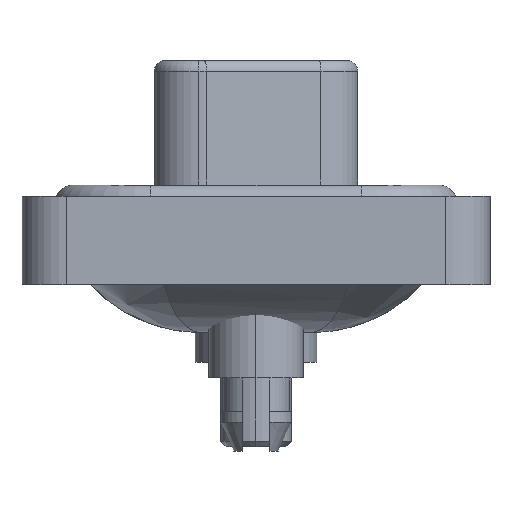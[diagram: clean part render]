
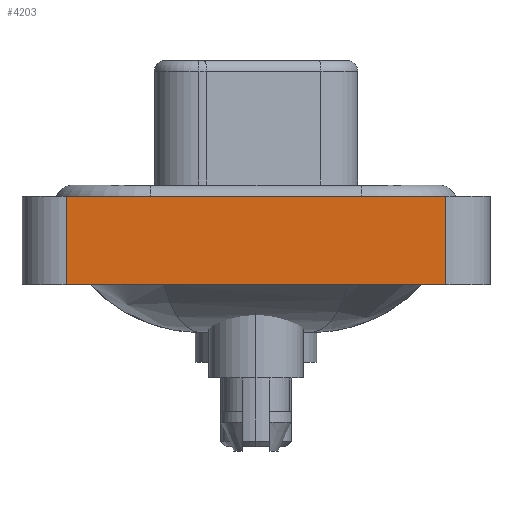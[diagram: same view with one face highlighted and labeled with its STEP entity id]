
A CAD part, left-side view. The second image highlights one B-rep face of the part: STEP entity #4203.
In plain terms, the highlighted planar face has unit normal (-1, 0, 0).
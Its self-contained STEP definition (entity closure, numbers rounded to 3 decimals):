
#140 = PLANE ( 'NONE',  #11697 ) ;
#316 = DIRECTION ( 'NONE',  ( 0., 0., 1. ) ) ;
#1077 = ORIENTED_EDGE ( 'NONE', *, *, #5960, .F. ) ;
#1085 = CARTESIAN_POINT ( 'NONE',  ( -7.3, -8.55, 0.4 ) ) ;
#1800 = VECTOR ( 'NONE', #1956, 1000. ) ;
#1956 = DIRECTION ( 'NONE',  ( 0., -1., 0. ) ) ;
#2335 = CARTESIAN_POINT ( 'NONE',  ( -7.3, -8.55, 0.4 ) ) ;
#3457 = EDGE_LOOP ( 'NONE', ( #10980, #4204, #1077, #15830 ) ) ;
#4203 = ADVANCED_FACE ( 'NONE', ( #16475 ), #140, .T. ) ;
#4204 = ORIENTED_EDGE ( 'NONE', *, *, #10672, .F. ) ;
#5868 = LINE ( 'NONE', #13966, #1800 ) ;
#5960 = EDGE_CURVE ( 'NONE', #15395, #13052, #7998, .T. ) ;
#6422 = DIRECTION ( 'NONE',  ( 0., -1., 0. ) ) ;
#6580 = CARTESIAN_POINT ( 'NONE',  ( -7.3, -8.55, -3.6 ) ) ;
#6786 = DIRECTION ( 'NONE',  ( -1., 0., 0. ) ) ;
#7095 = VERTEX_POINT ( 'NONE', #14334 ) ;
#7142 = CARTESIAN_POINT ( 'NONE',  ( -7.3, -8.55, -3.6 ) ) ;
#7898 = DIRECTION ( 'NONE',  ( 0., 0., 1. ) ) ;
#7998 = LINE ( 'NONE', #14607, #11193 ) ;
#9420 = EDGE_CURVE ( 'NONE', #7095, #11216, #14273, .T. ) ;
#9617 = EDGE_CURVE ( 'NONE', #15395, #7095, #5868, .T. ) ;
#10672 = EDGE_CURVE ( 'NONE', #13052, #11216, #13108, .T. ) ;
#10980 = ORIENTED_EDGE ( 'NONE', *, *, #9420, .T. ) ;
#11193 = VECTOR ( 'NONE', #11786, 1000. ) ;
#11216 = VERTEX_POINT ( 'NONE', #2335 ) ;
#11566 = VECTOR ( 'NONE', #6422, 1000. ) ;
#11697 = AXIS2_PLACEMENT_3D ( 'NONE', #7142, #6786, #316 ) ;
#11786 = DIRECTION ( 'NONE',  ( 0., 0., 1. ) ) ;
#13052 = VERTEX_POINT ( 'NONE', #16818 ) ;
#13108 = LINE ( 'NONE', #1085, #11566 ) ;
#13271 = VECTOR ( 'NONE', #7898, 1000. ) ;
#13966 = CARTESIAN_POINT ( 'NONE',  ( -7.3, -8.55, -3.6 ) ) ;
#14273 = LINE ( 'NONE', #6580, #13271 ) ;
#14334 = CARTESIAN_POINT ( 'NONE',  ( -7.3, -8.55, -3.6 ) ) ;
#14438 = CARTESIAN_POINT ( 'NONE',  ( -7.3, 8.55, -3.6 ) ) ;
#14607 = CARTESIAN_POINT ( 'NONE',  ( -7.3, 8.55, -3.6 ) ) ;
#15395 = VERTEX_POINT ( 'NONE', #14438 ) ;
#15830 = ORIENTED_EDGE ( 'NONE', *, *, #9617, .T. ) ;
#16475 = FACE_OUTER_BOUND ( 'NONE', #3457, .T. ) ;
#16818 = CARTESIAN_POINT ( 'NONE',  ( -7.3, 8.55, 0.4 ) ) ;
